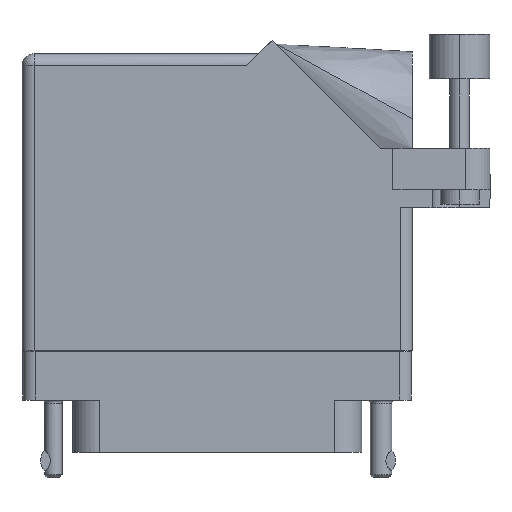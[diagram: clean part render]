
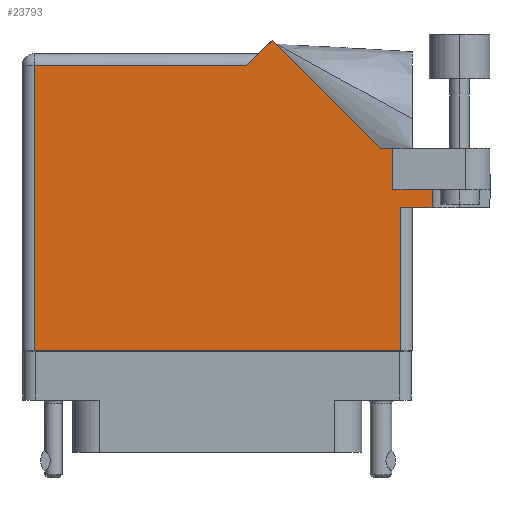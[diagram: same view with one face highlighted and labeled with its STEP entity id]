
A CAD part, front view. The second image highlights one B-rep face of the part: STEP entity #23793.
In plain terms, the highlighted face is planar.
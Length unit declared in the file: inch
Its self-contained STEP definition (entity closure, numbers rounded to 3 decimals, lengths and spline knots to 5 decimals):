
#370 = CARTESIAN_POINT ( 'NONE',  ( -0.943, -0.1, 0.455 ) ) ;
#643 = ORIENTED_EDGE ( 'NONE', *, *, #38590, .T. ) ;
#917 = LINE ( 'NONE', #36806, #40389 ) ;
#2512 = ORIENTED_EDGE ( 'NONE', *, *, #39407, .F. ) ;
#2742 = CARTESIAN_POINT ( 'NONE',  ( -1.005, 1.368, 0.455 ) ) ;
#3096 = VERTEX_POINT ( 'NONE', #33824 ) ;
#3542 = CARTESIAN_POINT ( 'NONE',  ( -1.005, -0.1, 0.455 ) ) ;
#4140 = DIRECTION ( 'NONE',  ( 1., 0., 0. ) ) ;
#4154 = EDGE_LOOP ( 'NONE', ( #40892, #16901, #34561, #24115, #2512, #643, #40025, #4866, #16096, #36282, #44874 ) ) ;
#4866 = ORIENTED_EDGE ( 'NONE', *, *, #12464, .T. ) ;
#7156 = VECTOR ( 'NONE', #11290, 39.37008 ) ;
#7334 = VECTOR ( 'NONE', #14476, 39.37008 ) ;
#7632 = FACE_OUTER_BOUND ( 'NONE', #4154, .T. ) ;
#7733 = VECTOR ( 'NONE', #13114, 39.37008 ) ;
#8603 = EDGE_CURVE ( 'NONE', #3096, #46750, #33473, .T. ) ;
#9765 = VERTEX_POINT ( 'NONE', #36155 ) ;
#10685 = VECTOR ( 'NONE', #22588, 39.37008 ) ;
#10790 = CARTESIAN_POINT ( 'NONE',  ( 0.212, 1.43, 0.455 ) ) ;
#11290 = DIRECTION ( 'NONE',  ( -0.707, -0.707, 0. ) ) ;
#11785 = VECTOR ( 'NONE', #30457, 39.37008 ) ;
#12464 = EDGE_CURVE ( 'NONE', #20174, #3096, #917, .T. ) ;
#13114 = DIRECTION ( 'NONE',  ( 0., -1., 0. ) ) ;
#13115 = VERTEX_POINT ( 'NONE', #17818 ) ;
#14101 = DIRECTION ( 'NONE',  ( -0.707, 0.707, 0. ) ) ;
#14476 = DIRECTION ( 'NONE',  ( -1., 0., 0. ) ) ;
#14707 = LINE ( 'NONE', #15365, #17113 ) ;
#15365 = CARTESIAN_POINT ( 'NONE',  ( 0.943, 0.637, 0.455 ) ) ;
#15696 = CARTESIAN_POINT ( 'NONE',  ( 1.1065, 1.06177, 0.455 ) ) ;
#16096 = ORIENTED_EDGE ( 'NONE', *, *, #8603, .T. ) ;
#16694 = PLANE ( 'NONE',  #40487 ) ;
#16857 = DIRECTION ( 'NONE',  ( 0., -1., 0. ) ) ;
#16901 = ORIENTED_EDGE ( 'NONE', *, *, #48379, .T. ) ;
#17113 = VECTOR ( 'NONE', #27151, 39.37008 ) ;
#17818 = CARTESIAN_POINT ( 'NONE',  ( -0.943, 1.368, 0.455 ) ) ;
#18537 = VERTEX_POINT ( 'NONE', #36823 ) ;
#18821 = CARTESIAN_POINT ( 'NONE',  ( 1.405, 0.944, 0.455 ) ) ;
#20174 = VERTEX_POINT ( 'NONE', #27637 ) ;
#21340 = VERTEX_POINT ( 'NONE', #44749 ) ;
#21500 = DIRECTION ( 'NONE',  ( -1., 0., 0. ) ) ;
#21664 = CARTESIAN_POINT ( 'NONE',  ( 0.905, 0.731, 0.455 ) ) ;
#22277 = EDGE_CURVE ( 'NONE', #13115, #36723, #29877, .T. ) ;
#22555 = EDGE_CURVE ( 'NONE', #36723, #34058, #38263, .T. ) ;
#22588 = DIRECTION ( 'NONE',  ( 1., 0., 0. ) ) ;
#23729 = LINE ( 'NONE', #18821, #11785 ) ;
#23793 = ADVANCED_FACE ( 'NONE', ( #7632 ), #16694, .F. ) ;
#24003 = DIRECTION ( 'NONE',  ( 0., 1., 0. ) ) ;
#24115 = ORIENTED_EDGE ( 'NONE', *, *, #39623, .F. ) ;
#27151 = DIRECTION ( 'NONE',  ( 0., 1., 0. ) ) ;
#27508 = VECTOR ( 'NONE', #4140, 39.37008 ) ;
#27637 = CARTESIAN_POINT ( 'NONE',  ( 0.83942, 0.944, 0.455 ) ) ;
#28142 = CARTESIAN_POINT ( 'NONE',  ( 0.905, 0.731, 0.455 ) ) ;
#28801 = CARTESIAN_POINT ( 'NONE',  ( -0.943, -0.1, 0.455 ) ) ;
#29822 = LINE ( 'NONE', #30104, #10685 ) ;
#29877 = LINE ( 'NONE', #28801, #7733 ) ;
#30081 = CARTESIAN_POINT ( 'NONE',  ( 0.15, 1.368, 0.455 ) ) ;
#30104 = CARTESIAN_POINT ( 'NONE',  ( 1.005, 0.637, 0.455 ) ) ;
#30457 = DIRECTION ( 'NONE',  ( -1., 0., 0. ) ) ;
#30506 = VECTOR ( 'NONE', #16857, 39.37008 ) ;
#31414 = EDGE_CURVE ( 'NONE', #46750, #13115, #36690, .T. ) ;
#32380 = CARTESIAN_POINT ( 'NONE',  ( 0.943, -0.1, 0.455 ) ) ;
#33473 = LINE ( 'NONE', #10790, #7156 ) ;
#33689 = CARTESIAN_POINT ( 'NONE',  ( 1.1065, 0.731, 0.455 ) ) ;
#33824 = CARTESIAN_POINT ( 'NONE',  ( 0.28271, 1.50071, 0.455 ) ) ;
#34058 = VERTEX_POINT ( 'NONE', #32380 ) ;
#34286 = VERTEX_POINT ( 'NONE', #33689 ) ;
#34561 = ORIENTED_EDGE ( 'NONE', *, *, #34751, .T. ) ;
#34751 = EDGE_CURVE ( 'NONE', #18537, #9765, #29822, .T. ) ;
#35896 = LINE ( 'NONE', #45995, #27508 ) ;
#36155 = CARTESIAN_POINT ( 'NONE',  ( 1.1065, 0.637, 0.455 ) ) ;
#36282 = ORIENTED_EDGE ( 'NONE', *, *, #31414, .T. ) ;
#36518 = LINE ( 'NONE', #15696, #30506 ) ;
#36690 = LINE ( 'NONE', #2742, #7334 ) ;
#36702 = DIRECTION ( 'NONE',  ( 0., 0., -1. ) ) ;
#36723 = VERTEX_POINT ( 'NONE', #370 ) ;
#36806 = CARTESIAN_POINT ( 'NONE',  ( 0.83942, 0.944, 0.455 ) ) ;
#36823 = CARTESIAN_POINT ( 'NONE',  ( 0.943, 0.637, 0.455 ) ) ;
#37903 = VERTEX_POINT ( 'NONE', #21664 ) ;
#37972 = DIRECTION ( 'NONE',  ( 1., 0., 0. ) ) ;
#38263 = LINE ( 'NONE', #3542, #43128 ) ;
#38590 = EDGE_CURVE ( 'NONE', #37903, #21340, #43822, .T. ) ;
#39407 = EDGE_CURVE ( 'NONE', #37903, #34286, #35896, .T. ) ;
#39623 = EDGE_CURVE ( 'NONE', #34286, #9765, #36518, .T. ) ;
#40025 = ORIENTED_EDGE ( 'NONE', *, *, #43027, .T. ) ;
#40389 = VECTOR ( 'NONE', #14101, 39.37008 ) ;
#40487 = AXIS2_PLACEMENT_3D ( 'NONE', #43793, #36702, #21500 ) ;
#40892 = ORIENTED_EDGE ( 'NONE', *, *, #22555, .T. ) ;
#43027 = EDGE_CURVE ( 'NONE', #21340, #20174, #23729, .T. ) ;
#43128 = VECTOR ( 'NONE', #37972, 39.37008 ) ;
#43793 = CARTESIAN_POINT ( 'NONE',  ( -1.005, 1.43, 0.455 ) ) ;
#43822 = LINE ( 'NONE', #28142, #44382 ) ;
#44382 = VECTOR ( 'NONE', #24003, 39.37008 ) ;
#44749 = CARTESIAN_POINT ( 'NONE',  ( 0.905, 0.944, 0.455 ) ) ;
#44874 = ORIENTED_EDGE ( 'NONE', *, *, #22277, .T. ) ;
#45995 = CARTESIAN_POINT ( 'NONE',  ( 0.905, 0.731, 0.455 ) ) ;
#46750 = VERTEX_POINT ( 'NONE', #30081 ) ;
#48379 = EDGE_CURVE ( 'NONE', #34058, #18537, #14707, .T. ) ;
